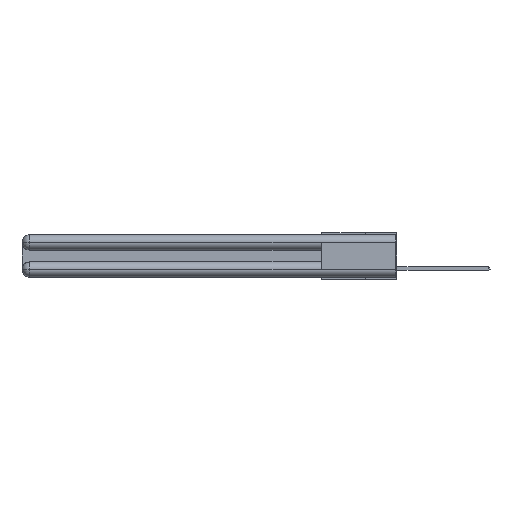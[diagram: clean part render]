
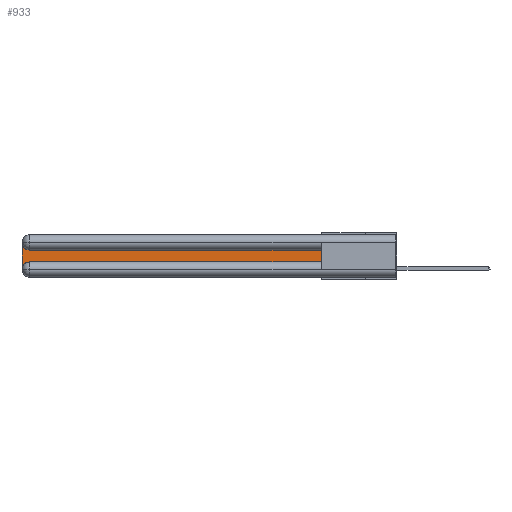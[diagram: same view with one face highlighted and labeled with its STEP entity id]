
A CAD part, left-side view. The second image highlights one B-rep face of the part: STEP entity #933.
In plain terms, the highlighted planar face has unit normal (-1, 0, 0).
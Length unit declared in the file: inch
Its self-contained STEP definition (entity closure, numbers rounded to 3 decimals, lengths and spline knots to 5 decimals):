
#33 = DIRECTION ( 'NONE',  ( 1., 0., 0. ) ) ;
#933 = ADVANCED_FACE ( 'NONE', ( #7465 ), #10462, .F. ) ;
#1154 = VERTEX_POINT ( 'NONE', #24469 ) ;
#1600 = AXIS2_PLACEMENT_3D ( 'NONE', #25742, #27946, #3938 ) ;
#1823 = LINE ( 'NONE', #19281, #24402 ) ;
#2512 = DIRECTION ( 'NONE',  ( 0., 0., -1. ) ) ;
#3320 = CARTESIAN_POINT ( 'NONE',  ( 0.075, 0.6, -0.1225 ) ) ;
#3638 = EDGE_CURVE ( 'NONE', #8405, #13014, #1823, .T. ) ;
#3938 = DIRECTION ( 'NONE',  ( 0., 0., -1. ) ) ;
#4379 = ORIENTED_EDGE ( 'NONE', *, *, #24290, .T. ) ;
#4438 = CARTESIAN_POINT ( 'NONE',  ( 0.075, 0.6, -0.2175 ) ) ;
#5403 = VERTEX_POINT ( 'NONE', #18811 ) ;
#5666 = DIRECTION ( 'NONE',  ( 0., 0., -1. ) ) ;
#5789 = VECTOR ( 'NONE', #14912, 39.37008 ) ;
#6899 = VERTEX_POINT ( 'NONE', #17979 ) ;
#7390 = CARTESIAN_POINT ( 'NONE',  ( 0.075, 0.6, -0.1225 ) ) ;
#7465 = FACE_OUTER_BOUND ( 'NONE', #23544, .T. ) ;
#8405 = VERTEX_POINT ( 'NONE', #12205 ) ;
#9632 = DIRECTION ( 'NONE',  ( 0., 0., -1. ) ) ;
#9960 = CARTESIAN_POINT ( 'NONE',  ( 0.075, 3., -0.2175 ) ) ;
#10054 = ORIENTED_EDGE ( 'NONE', *, *, #23116, .T. ) ;
#10462 = PLANE ( 'NONE',  #1600 ) ;
#11573 = DIRECTION ( 'NONE',  ( 1., 0., 0. ) ) ;
#11990 = AXIS2_PLACEMENT_3D ( 'NONE', #16056, #11573, #9632 ) ;
#12080 = EDGE_CURVE ( 'NONE', #6899, #8405, #14226, .T. ) ;
#12177 = ORIENTED_EDGE ( 'NONE', *, *, #12080, .T. ) ;
#12205 = CARTESIAN_POINT ( 'NONE',  ( 0.075, 2.94, -0.2175 ) ) ;
#12843 = VECTOR ( 'NONE', #5666, 39.37008 ) ;
#13014 = VERTEX_POINT ( 'NONE', #4438 ) ;
#13213 = EDGE_CURVE ( 'NONE', #16034, #5403, #25718, .T. ) ;
#13876 = ORIENTED_EDGE ( 'NONE', *, *, #27891, .T. ) ;
#14226 = CIRCLE ( 'NONE', #21675, 0.06 ) ;
#14912 = DIRECTION ( 'NONE',  ( 0., 0., 1. ) ) ;
#15396 = ORIENTED_EDGE ( 'NONE', *, *, #3638, .T. ) ;
#16034 = VERTEX_POINT ( 'NONE', #3320 ) ;
#16056 = CARTESIAN_POINT ( 'NONE',  ( 0.075, 2.94, -0.0625 ) ) ;
#17979 = CARTESIAN_POINT ( 'NONE',  ( 0.075, 3., -0.2775 ) ) ;
#18811 = CARTESIAN_POINT ( 'NONE',  ( 0.075, 2.94, -0.1225 ) ) ;
#19281 = CARTESIAN_POINT ( 'NONE',  ( 0.075, 0.6, -0.2175 ) ) ;
#19845 = LINE ( 'NONE', #25766, #5789 ) ;
#20712 = ORIENTED_EDGE ( 'NONE', *, *, #13213, .T. ) ;
#21675 = AXIS2_PLACEMENT_3D ( 'NONE', #21944, #33, #2512 ) ;
#21944 = CARTESIAN_POINT ( 'NONE',  ( 0.075, 2.94, -0.2775 ) ) ;
#22048 = LINE ( 'NONE', #9960, #12843 ) ;
#22656 = DIRECTION ( 'NONE',  ( 0., 1., 0. ) ) ;
#22959 = VECTOR ( 'NONE', #22656, 39.37008 ) ;
#23116 = EDGE_CURVE ( 'NONE', #5403, #1154, #26401, .T. ) ;
#23544 = EDGE_LOOP ( 'NONE', ( #20712, #10054, #13876, #12177, #15396, #4379 ) ) ;
#24290 = EDGE_CURVE ( 'NONE', #13014, #16034, #19845, .T. ) ;
#24402 = VECTOR ( 'NONE', #25739, 39.37008 ) ;
#24469 = CARTESIAN_POINT ( 'NONE',  ( 0.075, 3., -0.0625 ) ) ;
#25718 = LINE ( 'NONE', #7390, #22959 ) ;
#25739 = DIRECTION ( 'NONE',  ( 0., -1., 0. ) ) ;
#25742 = CARTESIAN_POINT ( 'NONE',  ( 0.075, 3., -0.1225 ) ) ;
#25766 = CARTESIAN_POINT ( 'NONE',  ( 0.075, 0.6, -0.2175 ) ) ;
#26401 = CIRCLE ( 'NONE', #11990, 0.06 ) ;
#27891 = EDGE_CURVE ( 'NONE', #1154, #6899, #22048, .T. ) ;
#27946 = DIRECTION ( 'NONE',  ( 1., 0., 0. ) ) ;
